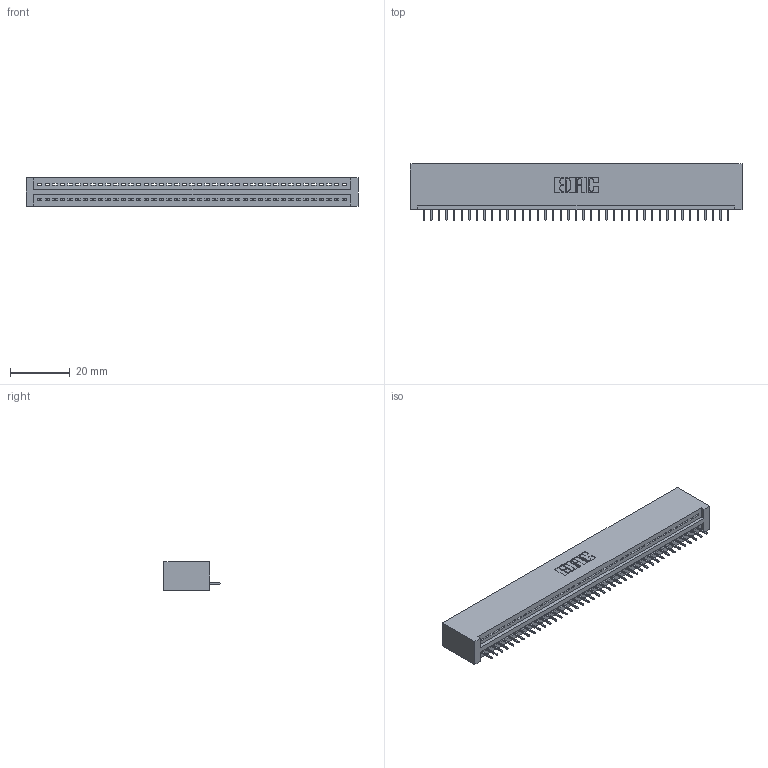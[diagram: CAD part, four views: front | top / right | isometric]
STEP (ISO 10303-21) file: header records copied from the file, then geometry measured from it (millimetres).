
FILE_DESCRIPTION (( 'STEP AP203' ), '1' );
FILE_NAME ('395-041-525-101.STEP', '2020-09-24T02:55:17', ( '' ), ( '' ), 'SwSTEP 2.0', 'SolidWorks 2020', '' );
FILE_SCHEMA (( 'CONFIG_CONTROL_DESIGN' ));
Length unit declared in the file: inch
Products named in the file (3): 345-292-001_345-293-125; 395-041-525-101; 345 Part_No Mounting Lugs
Assembly tree (42 placements, depth 2):
  395-041-525-101
    345 Part_No Mounting Lugs
    345-292-001_345-293-125  x41
Bounding box: 110.74 x 18.72 x 9.4 mm (x, y, z)
Volume: 10927.3 mm3; surface area: 14139.8 mm2
Topology: 42 solids, 42 shells, 2660 faces, 7697 edges, 4966 vertices
Faces by surface type: plane 1962, cylinder 698
Entity records: 30789 total; most frequent: CARTESIAN_POINT 5339, ORIENTED_EDGE 5314, DIRECTION 4659, EDGE_CURVE 2657, LINE 2373, VECTOR 2373, VERTEX_POINT 1766, AXIS2_PLACEMENT_3D 1143
